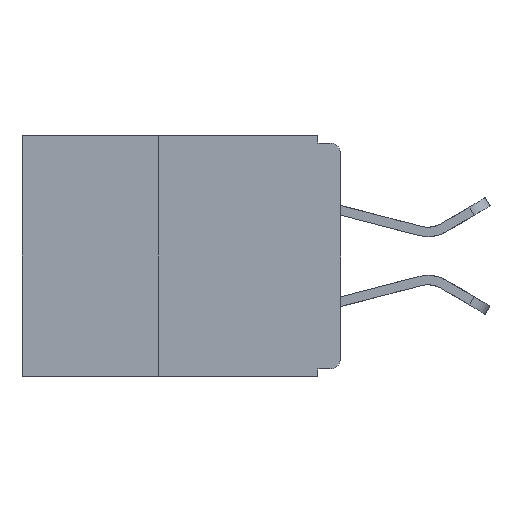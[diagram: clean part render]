
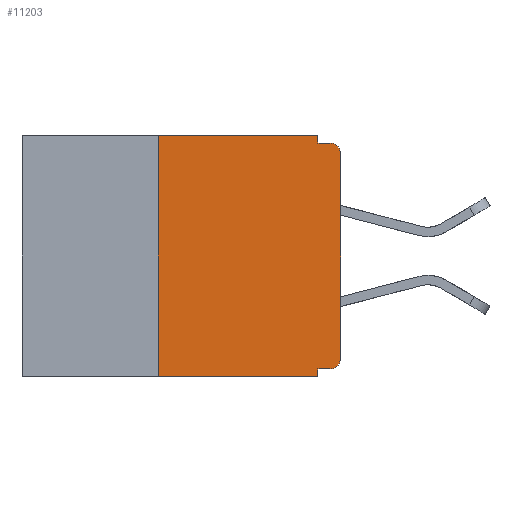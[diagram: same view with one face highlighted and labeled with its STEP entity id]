
A CAD part, left-side view. The second image highlights one B-rep face of the part: STEP entity #11203.
In plain terms, the highlighted planar face has unit normal (-1, 0, 0).
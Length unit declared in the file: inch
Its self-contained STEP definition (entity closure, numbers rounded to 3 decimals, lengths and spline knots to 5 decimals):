
#155 = ORIENTED_EDGE ( 'NONE', *, *, #15375, .F. ) ;
#226 = ORIENTED_EDGE ( 'NONE', *, *, #19849, .T. ) ;
#480 = CARTESIAN_POINT ( 'NONE',  ( 0., 0., -0.025 ) ) ;
#559 = ORIENTED_EDGE ( 'NONE', *, *, #10490, .F. ) ;
#1107 = CARTESIAN_POINT ( 'NONE',  ( 0., 0., 0. ) ) ;
#1136 = DIRECTION ( 'NONE',  ( 1., 0., 0. ) ) ;
#1275 = CARTESIAN_POINT ( 'NONE',  ( 0., 0.015, -0.32 ) ) ;
#1308 = CARTESIAN_POINT ( 'NONE',  ( 0., 0.015, -0.025 ) ) ;
#1559 = CARTESIAN_POINT ( 'NONE',  ( 0., 0.015, -0.305 ) ) ;
#2119 = CARTESIAN_POINT ( 'NONE',  ( 0., 0., -0.305 ) ) ;
#2229 = EDGE_CURVE ( 'NONE', #8806, #16842, #18256, .T. ) ;
#2240 = VECTOR ( 'NONE', #22197, 39.37008 ) ;
#2743 = AXIS2_PLACEMENT_3D ( 'NONE', #1559, #14356, #3420 ) ;
#2968 = VECTOR ( 'NONE', #9947, 39.37008 ) ;
#3165 = DIRECTION ( 'NONE',  ( 0., 0., -1. ) ) ;
#3420 = DIRECTION ( 'NONE',  ( 0., 0., -1. ) ) ;
#3731 = DIRECTION ( 'NONE',  ( 0., 0., -1. ) ) ;
#3790 = VECTOR ( 'NONE', #6575, 39.37008 ) ;
#3918 = VECTOR ( 'NONE', #8875, 39.37008 ) ;
#4102 = CARTESIAN_POINT ( 'NONE',  ( 0., 0.437, -0.33 ) ) ;
#4185 = DIRECTION ( 'NONE',  ( 0., -1., 0. ) ) ;
#4446 = CARTESIAN_POINT ( 'NONE',  ( 0., 0.031, 0. ) ) ;
#4672 = VECTOR ( 'NONE', #4185, 39.37008 ) ;
#5833 = VERTEX_POINT ( 'NONE', #480 ) ;
#6024 = ORIENTED_EDGE ( 'NONE', *, *, #23165, .F. ) ;
#6026 = AXIS2_PLACEMENT_3D ( 'NONE', #1308, #14106, #3165 ) ;
#6112 = EDGE_CURVE ( 'NONE', #14951, #5833, #6380, .T. ) ;
#6380 = LINE ( 'NONE', #1107, #19307 ) ;
#6575 = DIRECTION ( 'NONE',  ( 0., -1., 0. ) ) ;
#7037 = CARTESIAN_POINT ( 'NONE',  ( 0., 0.25, -0.33 ) ) ;
#7084 = ORIENTED_EDGE ( 'NONE', *, *, #14903, .F. ) ;
#7136 = CARTESIAN_POINT ( 'NONE',  ( 0., 0.031, -0.01 ) ) ;
#7268 = VERTEX_POINT ( 'NONE', #4446 ) ;
#7908 = CARTESIAN_POINT ( 'NONE',  ( 0., 0., -0.01 ) ) ;
#8421 = LINE ( 'NONE', #4102, #4672 ) ;
#8806 = VERTEX_POINT ( 'NONE', #7136 ) ;
#8875 = DIRECTION ( 'NONE',  ( 0., 0., -1. ) ) ;
#9184 = VECTOR ( 'NONE', #19625, 39.37008 ) ;
#9194 = CIRCLE ( 'NONE', #6026, 0.015 ) ;
#9633 = CARTESIAN_POINT ( 'NONE',  ( 0., 0.25, 0. ) ) ;
#9947 = DIRECTION ( 'NONE',  ( 0., 1., 0. ) ) ;
#10169 = LINE ( 'NONE', #17081, #2968 ) ;
#10490 = EDGE_CURVE ( 'NONE', #11797, #19497, #10169, .T. ) ;
#10929 = VERTEX_POINT ( 'NONE', #9633 ) ;
#11117 = CARTESIAN_POINT ( 'NONE',  ( 0., 0.031, 0. ) ) ;
#11203 = ADVANCED_FACE ( 'NONE', ( #15590 ), #12129, .F. ) ;
#11467 = LINE ( 'NONE', #11117, #19313 ) ;
#11797 = VERTEX_POINT ( 'NONE', #1275 ) ;
#12129 = PLANE ( 'NONE',  #16458 ) ;
#13278 = CARTESIAN_POINT ( 'NONE',  ( 0., 0.031, -0.32 ) ) ;
#13456 = EDGE_CURVE ( 'NONE', #18101, #21344, #8421, .T. ) ;
#13631 = LINE ( 'NONE', #19624, #3918 ) ;
#13908 = DIRECTION ( 'NONE',  ( 0., 0., 1. ) ) ;
#13916 = ORIENTED_EDGE ( 'NONE', *, *, #13456, .T. ) ;
#13933 = DIRECTION ( 'NONE',  ( 0., 0., -1. ) ) ;
#13978 = LINE ( 'NONE', #7037, #9184 ) ;
#14106 = DIRECTION ( 'NONE',  ( -1., 0., 0. ) ) ;
#14356 = DIRECTION ( 'NONE',  ( -1., 0., 0. ) ) ;
#14903 = EDGE_CURVE ( 'NONE', #7268, #8806, #11467, .T. ) ;
#14951 = VERTEX_POINT ( 'NONE', #2119 ) ;
#15375 = EDGE_CURVE ( 'NONE', #18101, #10929, #13978, .T. ) ;
#15590 = FACE_OUTER_BOUND ( 'NONE', #19798, .T. ) ;
#15650 = EDGE_CURVE ( 'NONE', #10929, #7268, #16759, .T. ) ;
#16458 = AXIS2_PLACEMENT_3D ( 'NONE', #19245, #1136, #13933 ) ;
#16759 = LINE ( 'NONE', #20409, #2240 ) ;
#16842 = VERTEX_POINT ( 'NONE', #17946 ) ;
#17081 = CARTESIAN_POINT ( 'NONE',  ( 0., 0., -0.32 ) ) ;
#17946 = CARTESIAN_POINT ( 'NONE',  ( 0., 0.015, -0.01 ) ) ;
#18101 = VERTEX_POINT ( 'NONE', #20494 ) ;
#18256 = LINE ( 'NONE', #7908, #3790 ) ;
#18319 = ORIENTED_EDGE ( 'NONE', *, *, #6112, .T. ) ;
#18416 = CARTESIAN_POINT ( 'NONE',  ( 0., 0.031, -0.33 ) ) ;
#18625 = ORIENTED_EDGE ( 'NONE', *, *, #2229, .F. ) ;
#19245 = CARTESIAN_POINT ( 'NONE',  ( 0., 0.437, 0. ) ) ;
#19307 = VECTOR ( 'NONE', #13908, 39.37008 ) ;
#19313 = VECTOR ( 'NONE', #3731, 39.37008 ) ;
#19497 = VERTEX_POINT ( 'NONE', #13278 ) ;
#19624 = CARTESIAN_POINT ( 'NONE',  ( 0., 0.031, -0.33 ) ) ;
#19625 = DIRECTION ( 'NONE',  ( 0., 0., 1. ) ) ;
#19798 = EDGE_LOOP ( 'NONE', ( #18319, #23036, #18625, #7084, #21996, #155, #13916, #6024, #559, #226 ) ) ;
#19849 = EDGE_CURVE ( 'NONE', #11797, #14951, #20833, .T. ) ;
#20409 = CARTESIAN_POINT ( 'NONE',  ( 0., 0.437, 0. ) ) ;
#20494 = CARTESIAN_POINT ( 'NONE',  ( 0., 0.25, -0.33 ) ) ;
#20833 = CIRCLE ( 'NONE', #2743, 0.015 ) ;
#21344 = VERTEX_POINT ( 'NONE', #18416 ) ;
#21996 = ORIENTED_EDGE ( 'NONE', *, *, #15650, .F. ) ;
#22197 = DIRECTION ( 'NONE',  ( 0., -1., 0. ) ) ;
#22489 = EDGE_CURVE ( 'NONE', #5833, #16842, #9194, .T. ) ;
#23036 = ORIENTED_EDGE ( 'NONE', *, *, #22489, .T. ) ;
#23165 = EDGE_CURVE ( 'NONE', #19497, #21344, #13631, .T. ) ;
